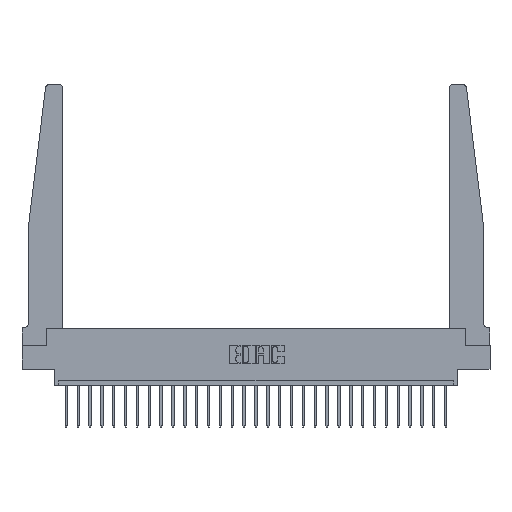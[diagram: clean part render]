
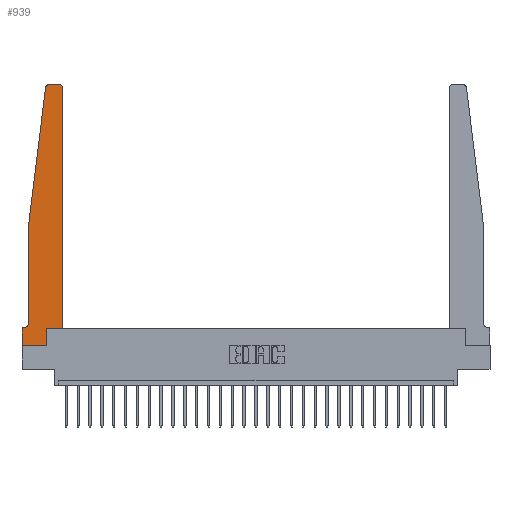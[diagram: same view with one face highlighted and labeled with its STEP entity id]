
A CAD part, top view. The second image highlights one B-rep face of the part: STEP entity #939.
In plain terms, the highlighted planar face has unit normal (0, 0, 1).
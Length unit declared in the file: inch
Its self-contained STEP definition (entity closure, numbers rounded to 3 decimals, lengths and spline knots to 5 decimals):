
#55 = ORIENTED_EDGE ( 'NONE', *, *, #21072, .T. ) ;
#939 = ADVANCED_FACE ( 'NONE', ( #1849 ), #1792, .T. ) ;
#1083 = CARTESIAN_POINT ( 'NONE',  ( 0.065, 1.25, 0.37 ) ) ;
#1296 = EDGE_CURVE ( 'NONE', #7758, #6436, #13459, .T. ) ;
#1475 = CARTESIAN_POINT ( 'NONE',  ( 0., 0.1875, 0.37 ) ) ;
#1486 = CARTESIAN_POINT ( 'NONE',  ( 0., 0., 0.37 ) ) ;
#1525 = VERTEX_POINT ( 'NONE', #1475 ) ;
#1577 = EDGE_CURVE ( 'NONE', #23358, #6082, #5347, .T. ) ;
#1792 = PLANE ( 'NONE',  #21643 ) ;
#1828 = DIRECTION ( 'NONE',  ( -0.122, -0.992, 0. ) ) ;
#1849 = FACE_OUTER_BOUND ( 'NONE', #3883, .T. ) ;
#2103 = LINE ( 'NONE', #8356, #22344 ) ;
#2332 = DIRECTION ( 'NONE',  ( 0., 1., 0. ) ) ;
#2367 = VERTEX_POINT ( 'NONE', #5506 ) ;
#2547 = CARTESIAN_POINT ( 'NONE',  ( 0.425, 2.72, 0.37 ) ) ;
#2603 = CARTESIAN_POINT ( 'NONE',  ( 0.395, 2.75, 0.37 ) ) ;
#2674 = ORIENTED_EDGE ( 'NONE', *, *, #1296, .T. ) ;
#3432 = CARTESIAN_POINT ( 'NONE',  ( 0.24675, 2.72367, 0.37 ) ) ;
#3840 = CARTESIAN_POINT ( 'NONE',  ( 0.065, 0.2375, 0.37 ) ) ;
#3883 = EDGE_LOOP ( 'NONE', ( #55, #18830, #13619, #21370, #5270, #21699, #16928, #4001, #2674, #16122, #20566, #14825 ) ) ;
#4001 = ORIENTED_EDGE ( 'NONE', *, *, #21010, .T. ) ;
#4033 = DIRECTION ( 'NONE',  ( 1., 0., 0. ) ) ;
#4297 = EDGE_CURVE ( 'NONE', #6436, #11767, #4548, .T. ) ;
#4548 = LINE ( 'NONE', #25354, #10413 ) ;
#5169 = CARTESIAN_POINT ( 'NONE',  ( 0.2605, 0., 0.37 ) ) ;
#5270 = ORIENTED_EDGE ( 'NONE', *, *, #22213, .T. ) ;
#5347 = LINE ( 'NONE', #7929, #10877 ) ;
#5506 = CARTESIAN_POINT ( 'NONE',  ( 0.27653, 2.75, 0.37 ) ) ;
#6080 = DIRECTION ( 'NONE',  ( 0., 0., -1. ) ) ;
#6082 = VERTEX_POINT ( 'NONE', #1083 ) ;
#6431 = DIRECTION ( 'NONE',  ( -1., 0., 0. ) ) ;
#6436 = VERTEX_POINT ( 'NONE', #14569 ) ;
#6940 = EDGE_CURVE ( 'NONE', #7473, #21217, #10905, .T. ) ;
#7074 = DIRECTION ( 'NONE',  ( 1., 0., 0. ) ) ;
#7473 = VERTEX_POINT ( 'NONE', #2547 ) ;
#7616 = EDGE_CURVE ( 'NONE', #16943, #1525, #24319, .T. ) ;
#7758 = VERTEX_POINT ( 'NONE', #5169 ) ;
#7929 = CARTESIAN_POINT ( 'NONE',  ( 0.065, 1.25, 0.37 ) ) ;
#8101 = CARTESIAN_POINT ( 'NONE',  ( 0.25, 2.75, 0.37 ) ) ;
#8263 = CARTESIAN_POINT ( 'NONE',  ( 0.015, 0.2375, 0.37 ) ) ;
#8286 = LINE ( 'NONE', #10022, #10580 ) ;
#8356 = CARTESIAN_POINT ( 'NONE',  ( 0.425, 0.18, 0.37 ) ) ;
#8951 = CARTESIAN_POINT ( 'NONE',  ( 0.065, 0.1875, 0.37 ) ) ;
#9130 = DIRECTION ( 'NONE',  ( -1., 0., 0. ) ) ;
#10022 = CARTESIAN_POINT ( 'NONE',  ( 0., 0., 0.37 ) ) ;
#10234 = VECTOR ( 'NONE', #23346, 39.37008 ) ;
#10413 = VECTOR ( 'NONE', #7074, 39.37008 ) ;
#10580 = VECTOR ( 'NONE', #4033, 39.37008 ) ;
#10877 = VECTOR ( 'NONE', #1828, 39.37008 ) ;
#10905 = CIRCLE ( 'NONE', #24887, 0.03 ) ;
#11146 = CARTESIAN_POINT ( 'NONE',  ( 0.2605, 0.18, 0.37 ) ) ;
#11432 = AXIS2_PLACEMENT_3D ( 'NONE', #15685, #15590, #21816 ) ;
#11767 = VERTEX_POINT ( 'NONE', #19368 ) ;
#13459 = LINE ( 'NONE', #11146, #10234 ) ;
#13619 = ORIENTED_EDGE ( 'NONE', *, *, #1577, .T. ) ;
#13686 = CIRCLE ( 'NONE', #16015, 0.05 ) ;
#13914 = CARTESIAN_POINT ( 'NONE',  ( 0.395, 2.72, 0.37 ) ) ;
#14569 = CARTESIAN_POINT ( 'NONE',  ( 0.2605, 0.18, 0.37 ) ) ;
#14726 = LINE ( 'NONE', #8101, #24040 ) ;
#14825 = ORIENTED_EDGE ( 'NONE', *, *, #6940, .T. ) ;
#15590 = DIRECTION ( 'NONE',  ( 0., 0., 1. ) ) ;
#15685 = CARTESIAN_POINT ( 'NONE',  ( 0.27653, 2.72, 0.37 ) ) ;
#15893 = DIRECTION ( 'NONE',  ( 0., -1., 0. ) ) ;
#16015 = AXIS2_PLACEMENT_3D ( 'NONE', #8263, #6080, #6431 ) ;
#16122 = ORIENTED_EDGE ( 'NONE', *, *, #4297, .T. ) ;
#16218 = CARTESIAN_POINT ( 'NONE',  ( 0., 0.1875, 0.37 ) ) ;
#16928 = ORIENTED_EDGE ( 'NONE', *, *, #20271, .T. ) ;
#16943 = VERTEX_POINT ( 'NONE', #26624 ) ;
#17919 = VECTOR ( 'NONE', #15893, 39.37008 ) ;
#18830 = ORIENTED_EDGE ( 'NONE', *, *, #23780, .T. ) ;
#19368 = CARTESIAN_POINT ( 'NONE',  ( 0.425, 0.18, 0.37 ) ) ;
#19789 = CARTESIAN_POINT ( 'NONE',  ( 0.065, 1.25, 0.37 ) ) ;
#20059 = DIRECTION ( 'NONE',  ( 0., -1., 0. ) ) ;
#20260 = EDGE_CURVE ( 'NONE', #6082, #22152, #23703, .T. ) ;
#20271 = EDGE_CURVE ( 'NONE', #1525, #25787, #20799, .T. ) ;
#20566 = ORIENTED_EDGE ( 'NONE', *, *, #22376, .T. ) ;
#20799 = LINE ( 'NONE', #1486, #17919 ) ;
#21010 = EDGE_CURVE ( 'NONE', #25787, #7758, #8286, .T. ) ;
#21072 = EDGE_CURVE ( 'NONE', #21217, #2367, #14726, .T. ) ;
#21217 = VERTEX_POINT ( 'NONE', #2603 ) ;
#21370 = ORIENTED_EDGE ( 'NONE', *, *, #20260, .T. ) ;
#21429 = VECTOR ( 'NONE', #20059, 39.37008 ) ;
#21643 = AXIS2_PLACEMENT_3D ( 'NONE', #16218, #26153, #26408 ) ;
#21699 = ORIENTED_EDGE ( 'NONE', *, *, #7616, .T. ) ;
#21722 = CARTESIAN_POINT ( 'NONE',  ( 0., 0., 0.37 ) ) ;
#21816 = DIRECTION ( 'NONE',  ( 1., 0., 0. ) ) ;
#22135 = DIRECTION ( 'NONE',  ( 0., 0., 1. ) ) ;
#22152 = VERTEX_POINT ( 'NONE', #3840 ) ;
#22213 = EDGE_CURVE ( 'NONE', #22152, #16943, #13686, .T. ) ;
#22344 = VECTOR ( 'NONE', #2332, 39.37008 ) ;
#22376 = EDGE_CURVE ( 'NONE', #11767, #7473, #2103, .T. ) ;
#22922 = CIRCLE ( 'NONE', #11432, 0.03 ) ;
#23346 = DIRECTION ( 'NONE',  ( 0., 1., 0. ) ) ;
#23358 = VERTEX_POINT ( 'NONE', #3432 ) ;
#23703 = LINE ( 'NONE', #19789, #21429 ) ;
#23780 = EDGE_CURVE ( 'NONE', #2367, #23358, #22922, .T. ) ;
#24040 = VECTOR ( 'NONE', #24569, 39.37008 ) ;
#24238 = DIRECTION ( 'NONE',  ( 1., 0., 0. ) ) ;
#24319 = LINE ( 'NONE', #8951, #25278 ) ;
#24569 = DIRECTION ( 'NONE',  ( -1., 0., 0. ) ) ;
#24887 = AXIS2_PLACEMENT_3D ( 'NONE', #13914, #22135, #24238 ) ;
#25278 = VECTOR ( 'NONE', #9130, 39.37008 ) ;
#25354 = CARTESIAN_POINT ( 'NONE',  ( 0.425, 0.18, 0.37 ) ) ;
#25787 = VERTEX_POINT ( 'NONE', #21722 ) ;
#26153 = DIRECTION ( 'NONE',  ( 0., 0., 1. ) ) ;
#26408 = DIRECTION ( 'NONE',  ( 1., 0., 0. ) ) ;
#26624 = CARTESIAN_POINT ( 'NONE',  ( 0.015, 0.1875, 0.37 ) ) ;
